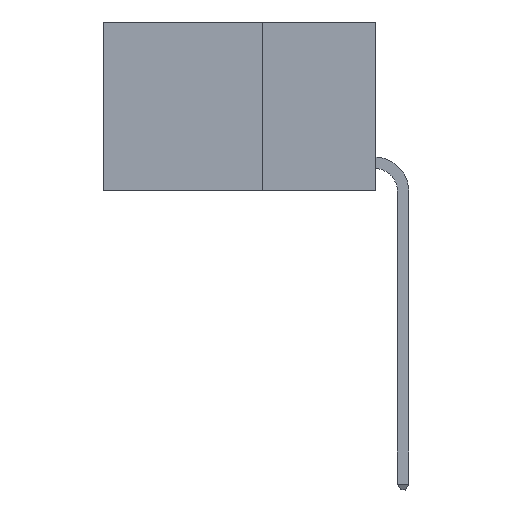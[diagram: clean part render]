
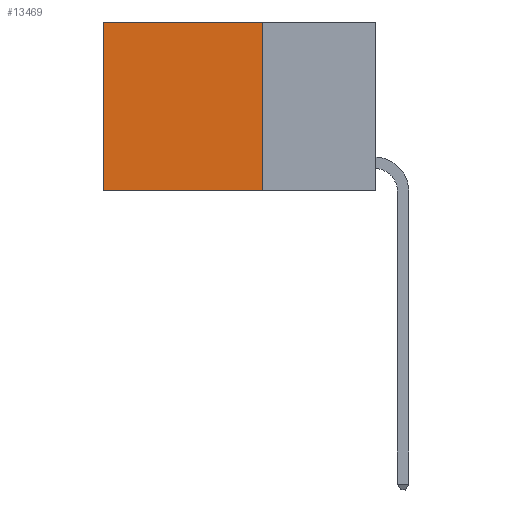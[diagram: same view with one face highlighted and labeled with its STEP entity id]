
A CAD part, left-side view. The second image highlights one B-rep face of the part: STEP entity #13469.
In plain terms, the highlighted planar face has unit normal (-1, 0, 0).
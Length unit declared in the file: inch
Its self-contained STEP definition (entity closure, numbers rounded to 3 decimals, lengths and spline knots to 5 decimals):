
#413 = VERTEX_POINT ( 'NONE', #19645 ) ;
#780 = VERTEX_POINT ( 'NONE', #3610 ) ;
#2626 = CARTESIAN_POINT ( 'NONE',  ( 0.2625, 0.25, 0. ) ) ;
#3229 = ORIENTED_EDGE ( 'NONE', *, *, #9299, .T. ) ;
#3536 = ORIENTED_EDGE ( 'NONE', *, *, #17339, .T. ) ;
#3564 = EDGE_LOOP ( 'NONE', ( #3229, #9263, #5992, #3536 ) ) ;
#3610 = CARTESIAN_POINT ( 'NONE',  ( 0.2625, 0.25, 0. ) ) ;
#3887 = DIRECTION ( 'NONE',  ( 0., 0., -1. ) ) ;
#4196 = VERTEX_POINT ( 'NONE', #5795 ) ;
#4363 = DIRECTION ( 'NONE',  ( 0., 0., -1. ) ) ;
#5213 = EDGE_CURVE ( 'NONE', #4196, #12596, #16348, .T. ) ;
#5795 = CARTESIAN_POINT ( 'NONE',  ( 0.2625, 0.25, -0.37 ) ) ;
#5992 = ORIENTED_EDGE ( 'NONE', *, *, #13784, .F. ) ;
#6397 = VECTOR ( 'NONE', #15715, 39.37008 ) ;
#7830 = VECTOR ( 'NONE', #3887, 39.37008 ) ;
#8249 = VECTOR ( 'NONE', #17362, 39.37008 ) ;
#8314 = LINE ( 'NONE', #9969, #7830 ) ;
#8364 = CARTESIAN_POINT ( 'NONE',  ( 0.2625, 0.6, -0.37 ) ) ;
#9263 = ORIENTED_EDGE ( 'NONE', *, *, #5213, .F. ) ;
#9299 = EDGE_CURVE ( 'NONE', #413, #12596, #8314, .T. ) ;
#9515 = CARTESIAN_POINT ( 'NONE',  ( 0.2625, 0.25, 0. ) ) ;
#9671 = CARTESIAN_POINT ( 'NONE',  ( 0.2625, 0.25, -0.37 ) ) ;
#9969 = CARTESIAN_POINT ( 'NONE',  ( 0.2625, 0.6, 0. ) ) ;
#10449 = PLANE ( 'NONE',  #14157 ) ;
#10454 = LINE ( 'NONE', #9515, #6397 ) ;
#11792 = DIRECTION ( 'NONE',  ( 0., 1., 0. ) ) ;
#12021 = CARTESIAN_POINT ( 'NONE',  ( 0.2625, 0.25, 0. ) ) ;
#12596 = VERTEX_POINT ( 'NONE', #8364 ) ;
#13136 = FACE_OUTER_BOUND ( 'NONE', #3564, .T. ) ;
#13469 = ADVANCED_FACE ( 'NONE', ( #13136 ), #10449, .F. ) ;
#13550 = DIRECTION ( 'NONE',  ( 1., 0., 0. ) ) ;
#13784 = EDGE_CURVE ( 'NONE', #780, #4196, #10454, .T. ) ;
#14122 = VECTOR ( 'NONE', #11792, 39.37008 ) ;
#14157 = AXIS2_PLACEMENT_3D ( 'NONE', #12021, #13550, #4363 ) ;
#14594 = LINE ( 'NONE', #2626, #14122 ) ;
#15715 = DIRECTION ( 'NONE',  ( 0., 0., -1. ) ) ;
#16348 = LINE ( 'NONE', #9671, #8249 ) ;
#17339 = EDGE_CURVE ( 'NONE', #780, #413, #14594, .T. ) ;
#17362 = DIRECTION ( 'NONE',  ( 0., 1., 0. ) ) ;
#19645 = CARTESIAN_POINT ( 'NONE',  ( 0.2625, 0.6, 0. ) ) ;
